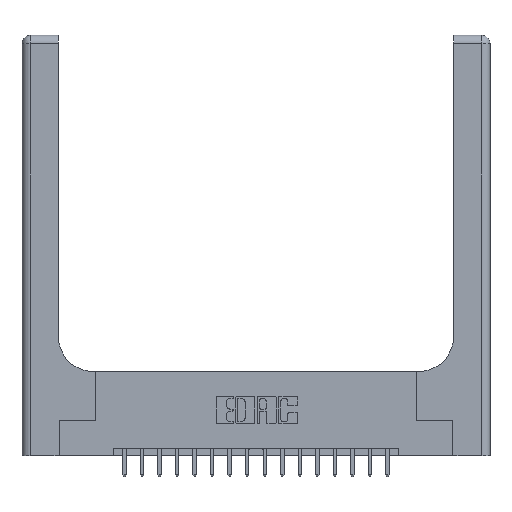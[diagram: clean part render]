
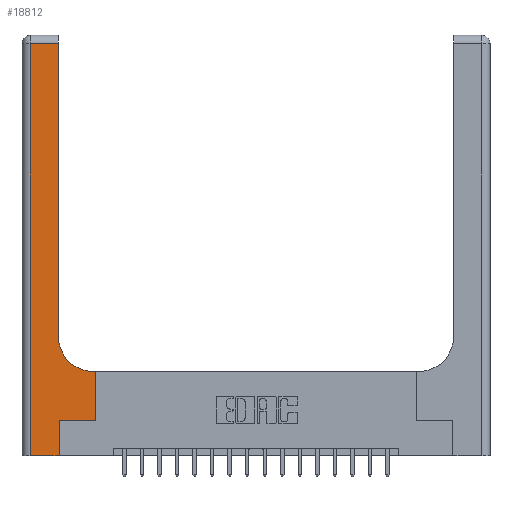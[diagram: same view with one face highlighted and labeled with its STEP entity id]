
A CAD part, top view. The second image highlights one B-rep face of the part: STEP entity #18812.
In plain terms, the highlighted planar face has unit normal (0, 0, 1).
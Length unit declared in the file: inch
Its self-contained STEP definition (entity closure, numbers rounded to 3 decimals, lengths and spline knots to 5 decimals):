
#498 = CARTESIAN_POINT ( 'NONE',  ( 0.26, 3., 0.37 ) ) ;
#504 = LINE ( 'NONE', #12898, #1414 ) ;
#545 = EDGE_CURVE ( 'NONE', #5741, #8947, #2766, .T. ) ;
#754 = LINE ( 'NONE', #18796, #6769 ) ;
#1262 = ORIENTED_EDGE ( 'NONE', *, *, #16449, .T. ) ;
#1407 = LINE ( 'NONE', #3182, #13630 ) ;
#1414 = VECTOR ( 'NONE', #4157, 39.37008 ) ;
#1506 = DIRECTION ( 'NONE',  ( 1., 0., 0. ) ) ;
#1700 = CARTESIAN_POINT ( 'NONE',  ( 0.51, 0.85, 0.37 ) ) ;
#1828 = DIRECTION ( 'NONE',  ( 0., 0., -1. ) ) ;
#2025 = DIRECTION ( 'NONE',  ( -1., 0., 0. ) ) ;
#2523 = CARTESIAN_POINT ( 'NONE',  ( 0.26, 0.6, 0.37 ) ) ;
#2620 = AXIS2_PLACEMENT_3D ( 'NONE', #1700, #10924, #1506 ) ;
#2766 = LINE ( 'NONE', #7329, #8865 ) ;
#3182 = CARTESIAN_POINT ( 'NONE',  ( 0.265, 0., 0.37 ) ) ;
#3950 = ORIENTED_EDGE ( 'NONE', *, *, #14937, .T. ) ;
#4157 = DIRECTION ( 'NONE',  ( 1., 0., 0. ) ) ;
#4481 = VERTEX_POINT ( 'NONE', #12014 ) ;
#4578 = EDGE_CURVE ( 'NONE', #4481, #8924, #504, .T. ) ;
#5176 = AXIS2_PLACEMENT_3D ( 'NONE', #16710, #1828, #2025 ) ;
#5304 = ORIENTED_EDGE ( 'NONE', *, *, #17209, .T. ) ;
#5372 = VERTEX_POINT ( 'NONE', #17755 ) ;
#5567 = EDGE_LOOP ( 'NONE', ( #5698, #1262, #6322, #3950, #8738, #11245, #12841, #5304, #15032 ) ) ;
#5698 = ORIENTED_EDGE ( 'NONE', *, *, #6280, .T. ) ;
#5741 = VERTEX_POINT ( 'NONE', #16394 ) ;
#6208 = VECTOR ( 'NONE', #12601, 39.37008 ) ;
#6280 = EDGE_CURVE ( 'NONE', #5372, #8272, #18930, .T. ) ;
#6322 = ORIENTED_EDGE ( 'NONE', *, *, #545, .T. ) ;
#6769 = VECTOR ( 'NONE', #17315, 39.37008 ) ;
#6969 = CARTESIAN_POINT ( 'NONE',  ( 0.528, 0.25, 0.37 ) ) ;
#7327 = VECTOR ( 'NONE', #12907, 39.37008 ) ;
#7329 = CARTESIAN_POINT ( 'NONE',  ( 0.06, 3., 0.37 ) ) ;
#7425 = DIRECTION ( 'NONE',  ( 0., -1., 0. ) ) ;
#7461 = DIRECTION ( 'NONE',  ( 0., 1., 0. ) ) ;
#7536 = CARTESIAN_POINT ( 'NONE',  ( 0.265, 0., 0.37 ) ) ;
#7610 = VERTEX_POINT ( 'NONE', #12187 ) ;
#7652 = DIRECTION ( 'NONE',  ( 1., 0., 0. ) ) ;
#8272 = VERTEX_POINT ( 'NONE', #14329 ) ;
#8445 = LINE ( 'NONE', #17655, #7327 ) ;
#8738 = ORIENTED_EDGE ( 'NONE', *, *, #14999, .T. ) ;
#8865 = VECTOR ( 'NONE', #7425, 39.37008 ) ;
#8924 = VERTEX_POINT ( 'NONE', #6969 ) ;
#8947 = VERTEX_POINT ( 'NONE', #14799 ) ;
#9047 = CARTESIAN_POINT ( 'NONE',  ( 0., 0., 0.37 ) ) ;
#9967 = LINE ( 'NONE', #2523, #16833 ) ;
#10763 = FACE_OUTER_BOUND ( 'NONE', #5567, .T. ) ;
#10924 = DIRECTION ( 'NONE',  ( 0., 0., -1. ) ) ;
#11057 = PLANE ( 'NONE',  #5176 ) ;
#11245 = ORIENTED_EDGE ( 'NONE', *, *, #4578, .T. ) ;
#12014 = CARTESIAN_POINT ( 'NONE',  ( 0.265, 0.25, 0.37 ) ) ;
#12187 = CARTESIAN_POINT ( 'NONE',  ( 0.528, 0.6, 0.37 ) ) ;
#12601 = DIRECTION ( 'NONE',  ( 0., 1., 0. ) ) ;
#12841 = ORIENTED_EDGE ( 'NONE', *, *, #18578, .T. ) ;
#12898 = CARTESIAN_POINT ( 'NONE',  ( 0.265, 0.25, 0.37 ) ) ;
#12907 = DIRECTION ( 'NONE',  ( -1., 0., 0. ) ) ;
#13308 = VECTOR ( 'NONE', #7652, 39.37008 ) ;
#13630 = VECTOR ( 'NONE', #7461, 39.37008 ) ;
#13756 = VERTEX_POINT ( 'NONE', #17041 ) ;
#14329 = CARTESIAN_POINT ( 'NONE',  ( 0.26, 2.94, 0.37 ) ) ;
#14721 = DIRECTION ( 'NONE',  ( -1., 0., 0. ) ) ;
#14799 = CARTESIAN_POINT ( 'NONE',  ( 0.06, 0., 0.37 ) ) ;
#14937 = EDGE_CURVE ( 'NONE', #8947, #15437, #17969, .T. ) ;
#14999 = EDGE_CURVE ( 'NONE', #15437, #4481, #1407, .T. ) ;
#15032 = ORIENTED_EDGE ( 'NONE', *, *, #17978, .T. ) ;
#15291 = CIRCLE ( 'NONE', #2620, 0.25 ) ;
#15437 = VERTEX_POINT ( 'NONE', #7536 ) ;
#16394 = CARTESIAN_POINT ( 'NONE',  ( 0.06, 2.94, 0.37 ) ) ;
#16449 = EDGE_CURVE ( 'NONE', #8272, #5741, #8445, .T. ) ;
#16710 = CARTESIAN_POINT ( 'NONE',  ( 0., 3., 0.37 ) ) ;
#16833 = VECTOR ( 'NONE', #14721, 39.37008 ) ;
#17041 = CARTESIAN_POINT ( 'NONE',  ( 0.51, 0.6, 0.37 ) ) ;
#17209 = EDGE_CURVE ( 'NONE', #7610, #13756, #9967, .T. ) ;
#17315 = DIRECTION ( 'NONE',  ( 0., 1., 0. ) ) ;
#17655 = CARTESIAN_POINT ( 'NONE',  ( 0., 2.94, 0.37 ) ) ;
#17755 = CARTESIAN_POINT ( 'NONE',  ( 0.26, 0.85, 0.37 ) ) ;
#17969 = LINE ( 'NONE', #9047, #13308 ) ;
#17978 = EDGE_CURVE ( 'NONE', #13756, #5372, #15291, .T. ) ;
#18578 = EDGE_CURVE ( 'NONE', #8924, #7610, #754, .T. ) ;
#18796 = CARTESIAN_POINT ( 'NONE',  ( 0.528, 0.25, 0.37 ) ) ;
#18812 = ADVANCED_FACE ( 'NONE', ( #10763 ), #11057, .F. ) ;
#18930 = LINE ( 'NONE', #498, #6208 ) ;
